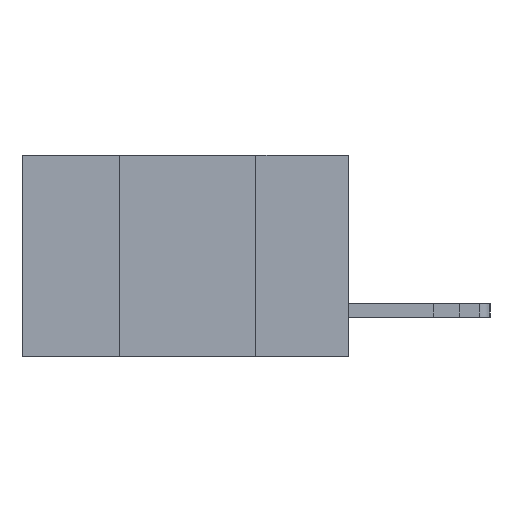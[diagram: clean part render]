
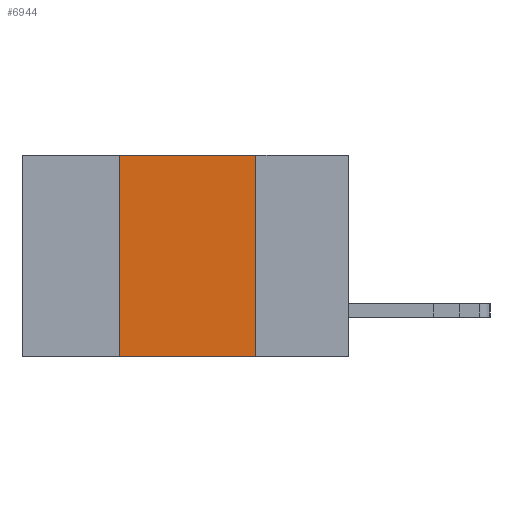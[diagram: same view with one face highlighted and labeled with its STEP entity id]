
A CAD part, left-side view. The second image highlights one B-rep face of the part: STEP entity #6944.
In plain terms, the highlighted planar face has unit normal (-1, 0, 0).
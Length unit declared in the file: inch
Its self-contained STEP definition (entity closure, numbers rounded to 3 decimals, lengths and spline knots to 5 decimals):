
#147 = FACE_OUTER_BOUND ( 'NONE', #8739, .T. ) ;
#175 = LINE ( 'NONE', #3255, #10308 ) ;
#208 = EDGE_CURVE ( 'NONE', #2826, #21949, #18741, .T. ) ;
#2390 = EDGE_CURVE ( 'NONE', #13681, #7634, #12762, .T. ) ;
#2660 = VECTOR ( 'NONE', #8068, 39.37008 ) ;
#2789 = VECTOR ( 'NONE', #3106, 39.37008 ) ;
#2826 = VERTEX_POINT ( 'NONE', #15834 ) ;
#3106 = DIRECTION ( 'NONE',  ( 0., 0., -1. ) ) ;
#3255 = CARTESIAN_POINT ( 'NONE',  ( 0., 0.6, -0.37 ) ) ;
#3359 = EDGE_CURVE ( 'NONE', #7634, #2826, #15446, .T. ) ;
#3617 = ORIENTED_EDGE ( 'NONE', *, *, #3359, .F. ) ;
#4643 = DIRECTION ( 'NONE',  ( 0., -1., 0. ) ) ;
#5101 = CARTESIAN_POINT ( 'NONE',  ( 0., 0.6, 0. ) ) ;
#5286 = DIRECTION ( 'NONE',  ( 0., -1., 0. ) ) ;
#6490 = EDGE_CURVE ( 'NONE', #13681, #21949, #175, .T. ) ;
#6633 = DIRECTION ( 'NONE',  ( 1., 0., 0. ) ) ;
#6896 = ORIENTED_EDGE ( 'NONE', *, *, #6490, .T. ) ;
#6944 = ADVANCED_FACE ( 'NONE', ( #147 ), #18538, .F. ) ;
#7090 = CARTESIAN_POINT ( 'NONE',  ( 0., 0.42, 0. ) ) ;
#7634 = VERTEX_POINT ( 'NONE', #14558 ) ;
#8068 = DIRECTION ( 'NONE',  ( 0., 0., 1. ) ) ;
#8739 = EDGE_LOOP ( 'NONE', ( #12516, #3617, #19856, #6896 ) ) ;
#10308 = VECTOR ( 'NONE', #5286, 39.37008 ) ;
#11337 = CARTESIAN_POINT ( 'NONE',  ( 0., 0.42, -0.37 ) ) ;
#12516 = ORIENTED_EDGE ( 'NONE', *, *, #208, .F. ) ;
#12762 = LINE ( 'NONE', #7090, #2660 ) ;
#13681 = VERTEX_POINT ( 'NONE', #11337 ) ;
#14558 = CARTESIAN_POINT ( 'NONE',  ( 0., 0.42, 0. ) ) ;
#15446 = LINE ( 'NONE', #5101, #20084 ) ;
#15834 = CARTESIAN_POINT ( 'NONE',  ( 0., 0.17, 0. ) ) ;
#16065 = CARTESIAN_POINT ( 'NONE',  ( 0., 0.17, -0.37 ) ) ;
#16535 = CARTESIAN_POINT ( 'NONE',  ( 0., 0.6, 0. ) ) ;
#18538 = PLANE ( 'NONE',  #20224 ) ;
#18741 = LINE ( 'NONE', #18939, #2789 ) ;
#18939 = CARTESIAN_POINT ( 'NONE',  ( 0., 0.17, 0. ) ) ;
#19856 = ORIENTED_EDGE ( 'NONE', *, *, #2390, .F. ) ;
#20084 = VECTOR ( 'NONE', #4643, 39.37008 ) ;
#20224 = AXIS2_PLACEMENT_3D ( 'NONE', #16535, #6633, #20488 ) ;
#20488 = DIRECTION ( 'NONE',  ( 0., 0., -1. ) ) ;
#21949 = VERTEX_POINT ( 'NONE', #16065 ) ;
